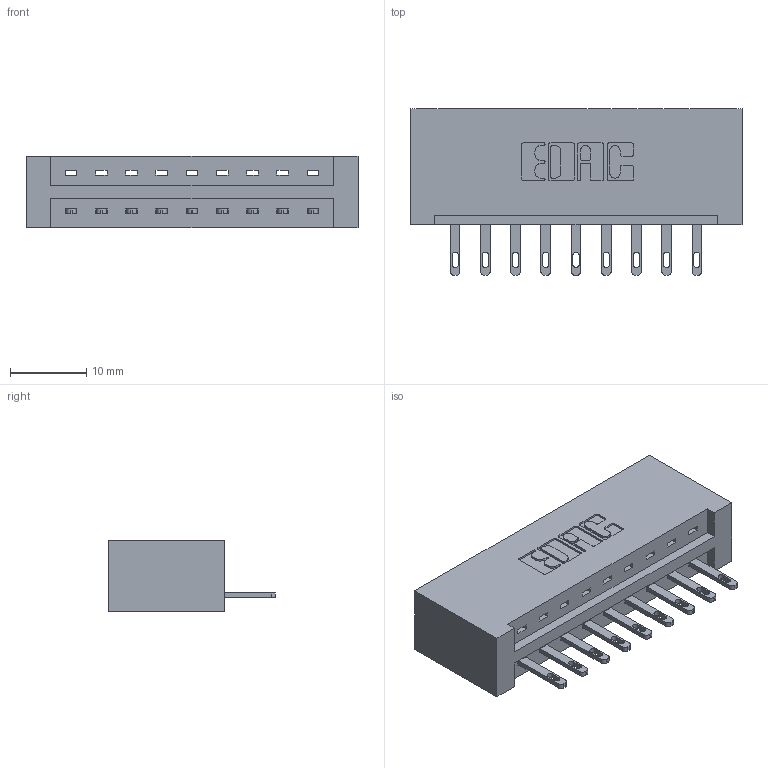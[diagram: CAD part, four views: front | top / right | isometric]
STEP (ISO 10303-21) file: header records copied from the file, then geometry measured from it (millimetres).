
FILE_DESCRIPTION (( 'STEP AP203' ), '1' );
FILE_NAME ('337-009-500-101.STEP', '2019-09-27T19:33:56', ( '' ), ( '' ), 'SwSTEP 2.0', 'SolidWorks 2016', '' );
FILE_SCHEMA (( 'CONFIG_CONTROL_DESIGN' ));
Length unit declared in the file: inch
Products named in the file (3): 337-009-500-101; 345-292-001_345-293-100; 337 Part_No Mounting Lugs
Assembly tree (10 placements, depth 2):
  337-009-500-101
    337 Part_No Mounting Lugs
    345-292-001_345-293-100  x9
Bounding box: 43.54 x 21.85 x 9.4 mm (x, y, z)
Volume: 4856.1 mm3; surface area: 4837.4 mm2
Topology: 10 solids, 10 shells, 628 faces, 1907 edges, 1270 vertices
Faces by surface type: plane 426, cylinder 202
Entity records: 10611 total; most frequent: CARTESIAN_POINT 1853, ORIENTED_EDGE 1798, DIRECTION 1621, EDGE_CURVE 899, VECTOR 775, LINE 775, VERTEX_POINT 598, AXIS2_PLACEMENT_3D 423
